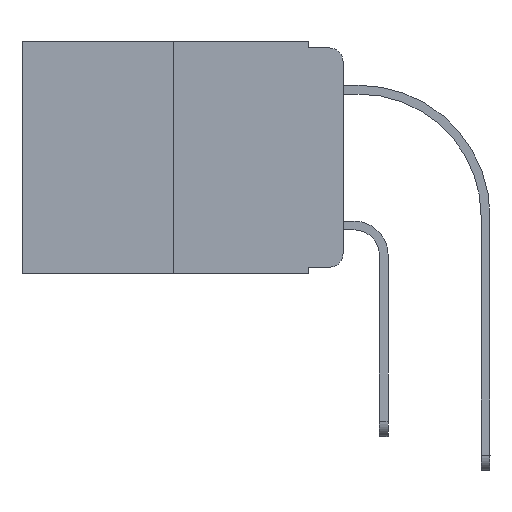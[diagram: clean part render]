
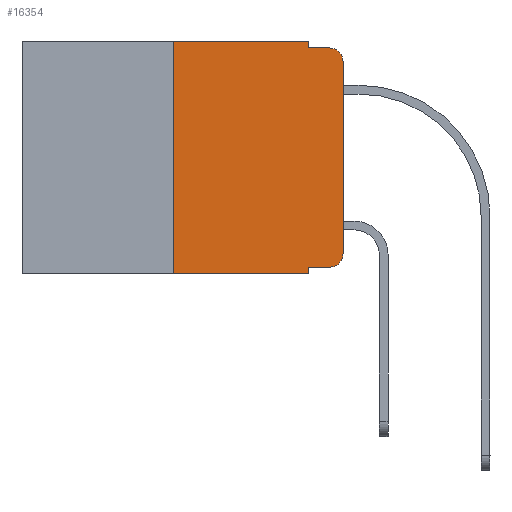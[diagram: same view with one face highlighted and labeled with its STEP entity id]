
A CAD part, left-side view. The second image highlights one B-rep face of the part: STEP entity #16354.
In plain terms, the highlighted planar face has unit normal (-1, 0, 0).
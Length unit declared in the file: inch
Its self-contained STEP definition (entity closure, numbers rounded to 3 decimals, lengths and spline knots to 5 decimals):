
#677 = VERTEX_POINT ( 'NONE', #13759 ) ;
#703 = CARTESIAN_POINT ( 'NONE',  ( 0., 0.25, 0. ) ) ;
#979 = VECTOR ( 'NONE', #5923, 39.37008 ) ;
#1220 = EDGE_CURVE ( 'NONE', #11461, #10356, #2917, .T. ) ;
#1538 = VECTOR ( 'NONE', #7812, 39.37008 ) ;
#1552 = CARTESIAN_POINT ( 'NONE',  ( 0., 0., -0.03 ) ) ;
#1559 = LINE ( 'NONE', #7030, #14491 ) ;
#1657 = CARTESIAN_POINT ( 'NONE',  ( 0., 0.051, -0.343 ) ) ;
#1837 = VERTEX_POINT ( 'NONE', #3257 ) ;
#1944 = ORIENTED_EDGE ( 'NONE', *, *, #4583, .T. ) ;
#1969 = LINE ( 'NONE', #703, #2724 ) ;
#2078 = VERTEX_POINT ( 'NONE', #4949 ) ;
#2173 = ORIENTED_EDGE ( 'NONE', *, *, #15571, .T. ) ;
#2290 = CARTESIAN_POINT ( 'NONE',  ( 0., 0., 0. ) ) ;
#2573 = CIRCLE ( 'NONE', #4589, 0.02 ) ;
#2583 = CARTESIAN_POINT ( 'NONE',  ( 0., 0.051, 0. ) ) ;
#2724 = VECTOR ( 'NONE', #15731, 39.37008 ) ;
#2904 = DIRECTION ( 'NONE',  ( 0., 0., -1. ) ) ;
#2917 = LINE ( 'NONE', #7038, #8276 ) ;
#3257 = CARTESIAN_POINT ( 'NONE',  ( 0., 0.25, 0. ) ) ;
#3399 = CARTESIAN_POINT ( 'NONE',  ( 0., 0., -0.313 ) ) ;
#4086 = ORIENTED_EDGE ( 'NONE', *, *, #8654, .F. ) ;
#4088 = DIRECTION ( 'NONE',  ( 0., 0., -1. ) ) ;
#4583 = EDGE_CURVE ( 'NONE', #16830, #17547, #9117, .T. ) ;
#4589 = AXIS2_PLACEMENT_3D ( 'NONE', #17151, #16977, #14273 ) ;
#4865 = EDGE_LOOP ( 'NONE', ( #1944, #2173, #10350, #10203, #17274, #4086, #5529, #11875, #16262, #13618 ) ) ;
#4949 = CARTESIAN_POINT ( 'NONE',  ( 0., 0.02, -0.01 ) ) ;
#4957 = EDGE_CURVE ( 'NONE', #5281, #16830, #6719, .T. ) ;
#4983 = DIRECTION ( 'NONE',  ( 0., -1., 0. ) ) ;
#5264 = VECTOR ( 'NONE', #14352, 39.37008 ) ;
#5281 = VERTEX_POINT ( 'NONE', #12932 ) ;
#5328 = FACE_OUTER_BOUND ( 'NONE', #4865, .T. ) ;
#5529 = ORIENTED_EDGE ( 'NONE', *, *, #11267, .T. ) ;
#5644 = VERTEX_POINT ( 'NONE', #14474 ) ;
#5692 = DIRECTION ( 'NONE',  ( -1., 0., 0. ) ) ;
#5923 = DIRECTION ( 'NONE',  ( 0., -1., 0. ) ) ;
#6019 = VECTOR ( 'NONE', #15268, 39.37008 ) ;
#6414 = CARTESIAN_POINT ( 'NONE',  ( 0., 0.473, 0. ) ) ;
#6719 = CIRCLE ( 'NONE', #9903, 0.02 ) ;
#6798 = CARTESIAN_POINT ( 'NONE',  ( 0., 0.25, -0.343 ) ) ;
#7026 = CARTESIAN_POINT ( 'NONE',  ( 0., 0.02, -0.313 ) ) ;
#7030 = CARTESIAN_POINT ( 'NONE',  ( 0., 0.051, -0.333 ) ) ;
#7038 = CARTESIAN_POINT ( 'NONE',  ( 0., 0.051, 0. ) ) ;
#7555 = CARTESIAN_POINT ( 'NONE',  ( 0., 0.051, -0.01 ) ) ;
#7812 = DIRECTION ( 'NONE',  ( 0., -1., 0. ) ) ;
#8104 = DIRECTION ( 'NONE',  ( 0., 0., -1. ) ) ;
#8276 = VECTOR ( 'NONE', #4088, 39.37008 ) ;
#8654 = EDGE_CURVE ( 'NONE', #16742, #1837, #1969, .T. ) ;
#9117 = LINE ( 'NONE', #2290, #5264 ) ;
#9227 = EDGE_CURVE ( 'NONE', #1837, #5644, #13341, .T. ) ;
#9401 = EDGE_CURVE ( 'NONE', #11461, #5281, #1559, .T. ) ;
#9453 = DIRECTION ( 'NONE',  ( 1., 0., 0. ) ) ;
#9903 = AXIS2_PLACEMENT_3D ( 'NONE', #7026, #5692, #2904 ) ;
#10203 = ORIENTED_EDGE ( 'NONE', *, *, #15470, .F. ) ;
#10350 = ORIENTED_EDGE ( 'NONE', *, *, #11001, .F. ) ;
#10356 = VERTEX_POINT ( 'NONE', #1657 ) ;
#10815 = PLANE ( 'NONE',  #10932 ) ;
#10932 = AXIS2_PLACEMENT_3D ( 'NONE', #16292, #9453, #8104 ) ;
#11001 = EDGE_CURVE ( 'NONE', #677, #2078, #17277, .T. ) ;
#11148 = LINE ( 'NONE', #12406, #979 ) ;
#11188 = DIRECTION ( 'NONE',  ( 0., -1., 0. ) ) ;
#11267 = EDGE_CURVE ( 'NONE', #16742, #10356, #11148, .T. ) ;
#11461 = VERTEX_POINT ( 'NONE', #14468 ) ;
#11875 = ORIENTED_EDGE ( 'NONE', *, *, #1220, .F. ) ;
#12406 = CARTESIAN_POINT ( 'NONE',  ( 0., 0.473, -0.343 ) ) ;
#12757 = VECTOR ( 'NONE', #4983, 39.37008 ) ;
#12932 = CARTESIAN_POINT ( 'NONE',  ( 0., 0.02, -0.333 ) ) ;
#13341 = LINE ( 'NONE', #6414, #12757 ) ;
#13618 = ORIENTED_EDGE ( 'NONE', *, *, #4957, .T. ) ;
#13641 = LINE ( 'NONE', #2583, #6019 ) ;
#13759 = CARTESIAN_POINT ( 'NONE',  ( 0., 0.051, -0.01 ) ) ;
#14273 = DIRECTION ( 'NONE',  ( 0., 0., -1. ) ) ;
#14352 = DIRECTION ( 'NONE',  ( 0., 0., 1. ) ) ;
#14468 = CARTESIAN_POINT ( 'NONE',  ( 0., 0.051, -0.333 ) ) ;
#14474 = CARTESIAN_POINT ( 'NONE',  ( 0., 0.051, 0. ) ) ;
#14491 = VECTOR ( 'NONE', #11188, 39.37008 ) ;
#15268 = DIRECTION ( 'NONE',  ( 0., 0., -1. ) ) ;
#15470 = EDGE_CURVE ( 'NONE', #5644, #677, #13641, .T. ) ;
#15571 = EDGE_CURVE ( 'NONE', #17547, #2078, #2573, .T. ) ;
#15731 = DIRECTION ( 'NONE',  ( 0., 0., 1. ) ) ;
#16262 = ORIENTED_EDGE ( 'NONE', *, *, #9401, .T. ) ;
#16292 = CARTESIAN_POINT ( 'NONE',  ( 0., 0.473, 0. ) ) ;
#16354 = ADVANCED_FACE ( 'NONE', ( #5328 ), #10815, .F. ) ;
#16742 = VERTEX_POINT ( 'NONE', #6798 ) ;
#16830 = VERTEX_POINT ( 'NONE', #3399 ) ;
#16977 = DIRECTION ( 'NONE',  ( -1., 0., 0. ) ) ;
#17151 = CARTESIAN_POINT ( 'NONE',  ( 0., 0.02, -0.03 ) ) ;
#17274 = ORIENTED_EDGE ( 'NONE', *, *, #9227, .F. ) ;
#17277 = LINE ( 'NONE', #7555, #1538 ) ;
#17547 = VERTEX_POINT ( 'NONE', #1552 ) ;
